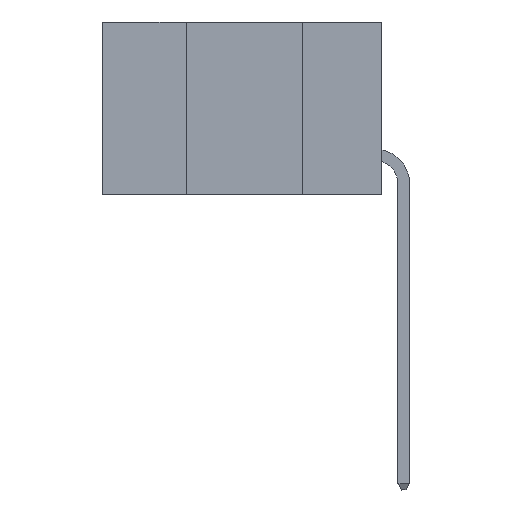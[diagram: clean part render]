
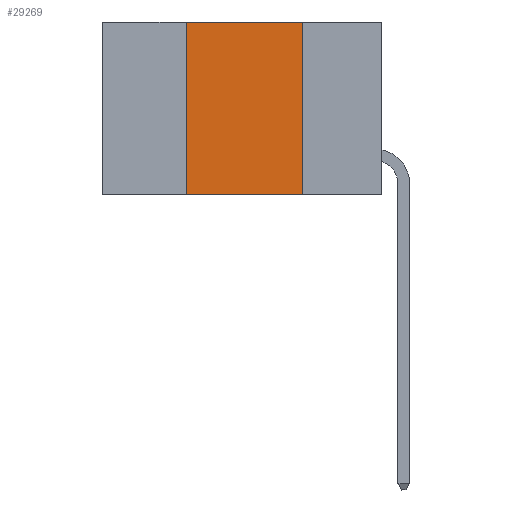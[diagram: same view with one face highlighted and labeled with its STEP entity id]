
A CAD part, left-side view. The second image highlights one B-rep face of the part: STEP entity #29269.
In plain terms, the highlighted planar face has unit normal (-1, 0, 0).
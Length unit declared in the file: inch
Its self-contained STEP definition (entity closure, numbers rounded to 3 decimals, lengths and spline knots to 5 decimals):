
#1647 = LINE ( 'NONE', #33283, #8233 ) ;
#3680 = VERTEX_POINT ( 'NONE', #43838 ) ;
#4293 = LINE ( 'NONE', #30886, #14719 ) ;
#6227 = EDGE_CURVE ( 'NONE', #20182, #36271, #1647, .T. ) ;
#7922 = DIRECTION ( 'NONE',  ( 0., 0., 1. ) ) ;
#8189 = EDGE_LOOP ( 'NONE', ( #38052, #13664, #32543, #42886 ) ) ;
#8233 = VECTOR ( 'NONE', #40160, 39.37008 ) ;
#13069 = DIRECTION ( 'NONE',  ( 0., -1., 0. ) ) ;
#13664 = ORIENTED_EDGE ( 'NONE', *, *, #35981, .F. ) ;
#14719 = VECTOR ( 'NONE', #20020, 39.37008 ) ;
#19333 = VECTOR ( 'NONE', #7922, 39.37008 ) ;
#19802 = CARTESIAN_POINT ( 'NONE',  ( 0., 0.6, 0. ) ) ;
#19881 = FACE_OUTER_BOUND ( 'NONE', #8189, .T. ) ;
#20020 = DIRECTION ( 'NONE',  ( 0., 0., -1. ) ) ;
#20182 = VERTEX_POINT ( 'NONE', #29847 ) ;
#23054 = VECTOR ( 'NONE', #13069, 39.37008 ) ;
#25724 = EDGE_CURVE ( 'NONE', #20182, #43360, #28683, .T. ) ;
#26835 = CARTESIAN_POINT ( 'NONE',  ( 0., 0.6, 0. ) ) ;
#28369 = CARTESIAN_POINT ( 'NONE',  ( 0., 0.17, -0.37 ) ) ;
#28649 = CARTESIAN_POINT ( 'NONE',  ( 0., 0.42, 0. ) ) ;
#28683 = LINE ( 'NONE', #28649, #19333 ) ;
#28960 = CARTESIAN_POINT ( 'NONE',  ( 0., 0.42, 0. ) ) ;
#29269 = ADVANCED_FACE ( 'NONE', ( #19881 ), #37258, .F. ) ;
#29847 = CARTESIAN_POINT ( 'NONE',  ( 0., 0.42, -0.37 ) ) ;
#30377 = DIRECTION ( 'NONE',  ( 1., 0., 0. ) ) ;
#30886 = CARTESIAN_POINT ( 'NONE',  ( 0., 0.17, 0. ) ) ;
#32381 = LINE ( 'NONE', #26835, #23054 ) ;
#32543 = ORIENTED_EDGE ( 'NONE', *, *, #25724, .F. ) ;
#33283 = CARTESIAN_POINT ( 'NONE',  ( 0., 0.6, -0.37 ) ) ;
#35981 = EDGE_CURVE ( 'NONE', #43360, #3680, #32381, .T. ) ;
#36271 = VERTEX_POINT ( 'NONE', #28369 ) ;
#37206 = EDGE_CURVE ( 'NONE', #3680, #36271, #4293, .T. ) ;
#37258 = PLANE ( 'NONE',  #39090 ) ;
#38052 = ORIENTED_EDGE ( 'NONE', *, *, #37206, .F. ) ;
#39090 = AXIS2_PLACEMENT_3D ( 'NONE', #19802, #30377, #44005 ) ;
#40160 = DIRECTION ( 'NONE',  ( 0., -1., 0. ) ) ;
#42886 = ORIENTED_EDGE ( 'NONE', *, *, #6227, .T. ) ;
#43360 = VERTEX_POINT ( 'NONE', #28960 ) ;
#43838 = CARTESIAN_POINT ( 'NONE',  ( 0., 0.17, 0. ) ) ;
#44005 = DIRECTION ( 'NONE',  ( 0., 0., -1. ) ) ;
